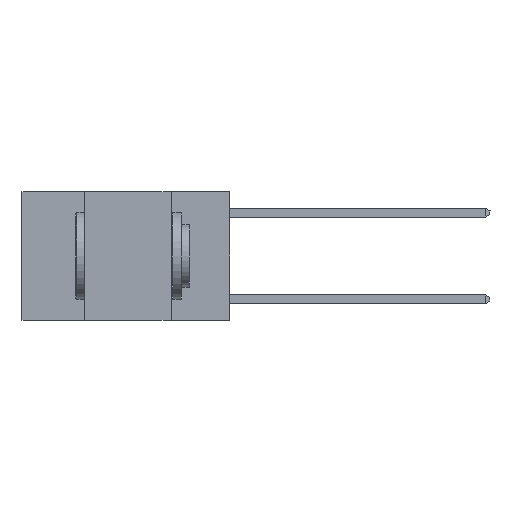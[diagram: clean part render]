
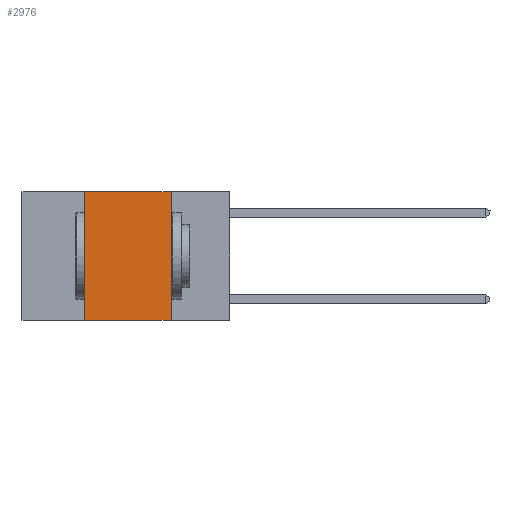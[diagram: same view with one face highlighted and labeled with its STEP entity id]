
A CAD part, left-side view. The second image highlights one B-rep face of the part: STEP entity #2976.
In plain terms, the highlighted planar face has unit normal (-1, 0, 0).
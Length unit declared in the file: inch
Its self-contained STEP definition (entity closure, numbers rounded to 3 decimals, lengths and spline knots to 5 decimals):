
#255 = EDGE_CURVE ( 'NONE', #7441, #4933, #8816, .T. ) ;
#500 = ORIENTED_EDGE ( 'NONE', *, *, #10094, .F. ) ;
#509 = VERTEX_POINT ( 'NONE', #5118 ) ;
#515 = PLANE ( 'NONE',  #6845 ) ;
#568 = DIRECTION ( 'NONE',  ( 0., 0., 1. ) ) ;
#682 = CARTESIAN_POINT ( 'NONE',  ( 0., 0.6, 0. ) ) ;
#1359 = DIRECTION ( 'NONE',  ( 0., -1., 0. ) ) ;
#1706 = LINE ( 'NONE', #8726, #3608 ) ;
#2522 = EDGE_LOOP ( 'NONE', ( #500, #7738, #5640, #8028 ) ) ;
#2976 = ADVANCED_FACE ( 'NONE', ( #8232 ), #515, .F. ) ;
#3608 = VECTOR ( 'NONE', #5150, 39.37008 ) ;
#3862 = VECTOR ( 'NONE', #6764, 39.37008 ) ;
#4173 = EDGE_CURVE ( 'NONE', #509, #5412, #1706, .T. ) ;
#4933 = VERTEX_POINT ( 'NONE', #6251 ) ;
#5118 = CARTESIAN_POINT ( 'NONE',  ( 0., 0.42, 0. ) ) ;
#5142 = CARTESIAN_POINT ( 'NONE',  ( 0., 0.42, 0. ) ) ;
#5150 = DIRECTION ( 'NONE',  ( 0., -1., 0. ) ) ;
#5412 = VERTEX_POINT ( 'NONE', #6166 ) ;
#5640 = ORIENTED_EDGE ( 'NONE', *, *, #10855, .F. ) ;
#5880 = CARTESIAN_POINT ( 'NONE',  ( 0., 0.17, 0. ) ) ;
#6166 = CARTESIAN_POINT ( 'NONE',  ( 0., 0.17, 0. ) ) ;
#6251 = CARTESIAN_POINT ( 'NONE',  ( 0., 0.17, -0.37 ) ) ;
#6330 = VECTOR ( 'NONE', #568, 39.37008 ) ;
#6438 = VECTOR ( 'NONE', #1359, 39.37008 ) ;
#6708 = CARTESIAN_POINT ( 'NONE',  ( 0., 0.42, -0.37 ) ) ;
#6764 = DIRECTION ( 'NONE',  ( 0., 0., -1. ) ) ;
#6845 = AXIS2_PLACEMENT_3D ( 'NONE', #682, #9439, #8133 ) ;
#7317 = CARTESIAN_POINT ( 'NONE',  ( 0., 0.6, -0.37 ) ) ;
#7441 = VERTEX_POINT ( 'NONE', #6708 ) ;
#7738 = ORIENTED_EDGE ( 'NONE', *, *, #4173, .F. ) ;
#7889 = LINE ( 'NONE', #5142, #6330 ) ;
#8028 = ORIENTED_EDGE ( 'NONE', *, *, #255, .T. ) ;
#8133 = DIRECTION ( 'NONE',  ( 0., 0., -1. ) ) ;
#8232 = FACE_OUTER_BOUND ( 'NONE', #2522, .T. ) ;
#8726 = CARTESIAN_POINT ( 'NONE',  ( 0., 0.6, 0. ) ) ;
#8816 = LINE ( 'NONE', #7317, #6438 ) ;
#8859 = LINE ( 'NONE', #5880, #3862 ) ;
#9439 = DIRECTION ( 'NONE',  ( 1., 0., 0. ) ) ;
#10094 = EDGE_CURVE ( 'NONE', #5412, #4933, #8859, .T. ) ;
#10855 = EDGE_CURVE ( 'NONE', #7441, #509, #7889, .T. ) ;
